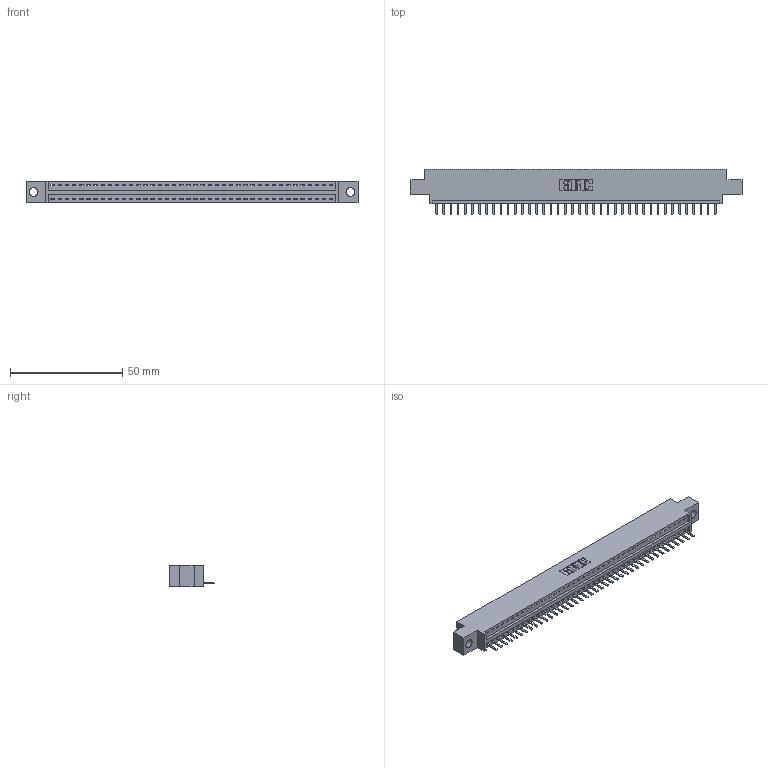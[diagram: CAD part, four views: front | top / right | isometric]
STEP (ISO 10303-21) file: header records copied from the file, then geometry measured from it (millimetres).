
FILE_DESCRIPTION (( 'STEP AP203' ), '1' );
FILE_NAME ('346-040-520-604.STEP', '2022-05-07T08:45:11', ( '' ), ( '' ), 'SwSTEP 2.0', 'SolidWorks 2020', '' );
FILE_SCHEMA (( 'CONFIG_CONTROL_DESIGN' ));
Length unit declared in the file: inch
Products named in the file (3): 346 Part_0.170 Offset - 0.156 Dia-TH; 345-292-001_345-293-120; 346-040-520-604
Assembly tree (41 placements, depth 2):
  346-040-520-604
    346 Part_0.170 Offset - 0.156 Dia-TH
    345-292-001_345-293-120  x40
Bounding box: 147.57 x 20.02 x 9.4 mm (x, y, z)
Volume: 13736.7 mm3; surface area: 16761 mm2
Topology: 41 solids, 41 shells, 2620 faces, 7737 edges, 5050 vertices
Faces by surface type: plane 1774, cylinder 846
Entity records: 25759 total; most frequent: CARTESIAN_POINT 4438, ORIENTED_EDGE 4398, DIRECTION 3903, EDGE_CURVE 2199, LINE 1903, VECTOR 1903, VERTEX_POINT 1462, AXIS2_PLACEMENT_3D 1000
